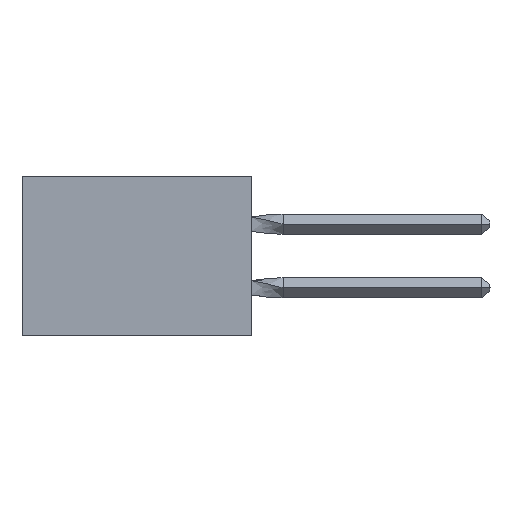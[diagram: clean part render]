
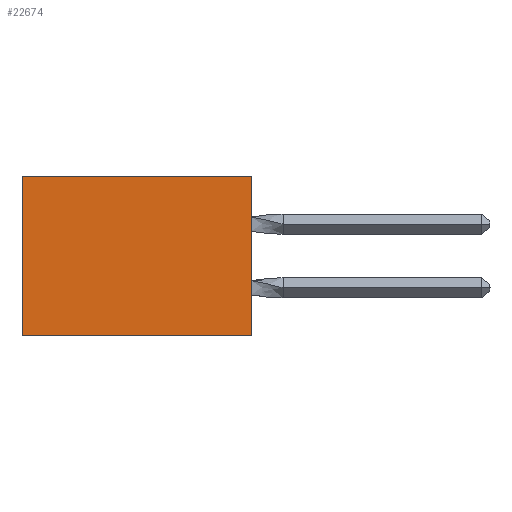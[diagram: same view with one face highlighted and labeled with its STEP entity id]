
A CAD part, left-side view. The second image highlights one B-rep face of the part: STEP entity #22674.
In plain terms, the highlighted planar face has unit normal (-1, 0, 0).
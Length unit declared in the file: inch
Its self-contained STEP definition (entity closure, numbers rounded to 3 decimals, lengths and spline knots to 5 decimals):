
#584 = DIRECTION ( 'NONE',  ( 0., 0., -1. ) ) ;
#650 = DIRECTION ( 'NONE',  ( 0., 1., 0. ) ) ;
#1211 = DIRECTION ( 'NONE',  ( 1., 0., 0. ) ) ;
#1725 = CARTESIAN_POINT ( 'NONE',  ( 0.305, 0., -0.5 ) ) ;
#2545 = DIRECTION ( 'NONE',  ( 0., 1., 0. ) ) ;
#3154 = EDGE_CURVE ( 'NONE', #22109, #17375, #24323, .T. ) ;
#3371 = VECTOR ( 'NONE', #584, 39.37008 ) ;
#3464 = DIRECTION ( 'NONE',  ( 0., 0., -1. ) ) ;
#4075 = EDGE_LOOP ( 'NONE', ( #26294, #5390, #10598, #6800 ) ) ;
#5390 = ORIENTED_EDGE ( 'NONE', *, *, #3154, .F. ) ;
#5709 = PLANE ( 'NONE',  #22505 ) ;
#6800 = ORIENTED_EDGE ( 'NONE', *, *, #16898, .T. ) ;
#8452 = DIRECTION ( 'NONE',  ( 0., 0., -1. ) ) ;
#10364 = VECTOR ( 'NONE', #2545, 39.37008 ) ;
#10410 = CARTESIAN_POINT ( 'NONE',  ( 0.305, 0.72, 0. ) ) ;
#10598 = ORIENTED_EDGE ( 'NONE', *, *, #15694, .F. ) ;
#13143 = CARTESIAN_POINT ( 'NONE',  ( 0.305, 0., 0. ) ) ;
#13997 = CARTESIAN_POINT ( 'NONE',  ( 0.305, 0.72, -0.5 ) ) ;
#14007 = CARTESIAN_POINT ( 'NONE',  ( 0.305, 0., 0. ) ) ;
#14062 = CARTESIAN_POINT ( 'NONE',  ( 0.305, 0., -0.5 ) ) ;
#15694 = EDGE_CURVE ( 'NONE', #22933, #22109, #26217, .T. ) ;
#16840 = CARTESIAN_POINT ( 'NONE',  ( 0.305, 0., -0.5 ) ) ;
#16898 = EDGE_CURVE ( 'NONE', #22933, #27189, #27268, .T. ) ;
#17375 = VERTEX_POINT ( 'NONE', #13997 ) ;
#19267 = VECTOR ( 'NONE', #650, 39.37008 ) ;
#20144 = CARTESIAN_POINT ( 'NONE',  ( 0.305, 0., -0.5 ) ) ;
#20887 = FACE_OUTER_BOUND ( 'NONE', #4075, .T. ) ;
#22109 = VERTEX_POINT ( 'NONE', #20144 ) ;
#22505 = AXIS2_PLACEMENT_3D ( 'NONE', #16840, #1211, #3464 ) ;
#22674 = ADVANCED_FACE ( 'NONE', ( #20887 ), #5709, .F. ) ;
#22750 = CARTESIAN_POINT ( 'NONE',  ( 0.305, 0.72, -0.5 ) ) ;
#22933 = VERTEX_POINT ( 'NONE', #13143 ) ;
#23319 = EDGE_CURVE ( 'NONE', #27189, #17375, #26741, .T. ) ;
#24323 = LINE ( 'NONE', #14062, #10364 ) ;
#25525 = VECTOR ( 'NONE', #8452, 39.37008 ) ;
#26217 = LINE ( 'NONE', #1725, #25525 ) ;
#26294 = ORIENTED_EDGE ( 'NONE', *, *, #23319, .T. ) ;
#26741 = LINE ( 'NONE', #22750, #3371 ) ;
#27189 = VERTEX_POINT ( 'NONE', #10410 ) ;
#27268 = LINE ( 'NONE', #14007, #19267 ) ;
